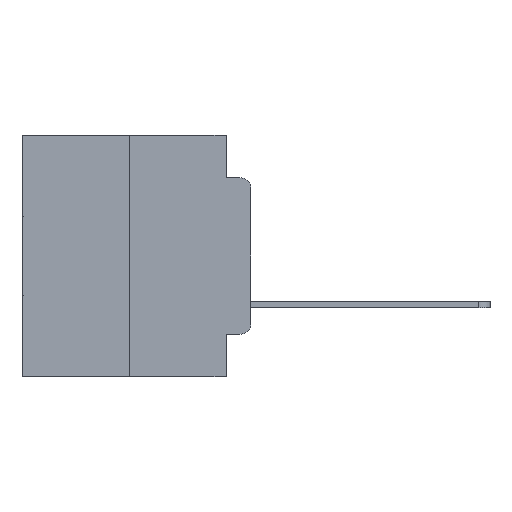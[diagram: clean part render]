
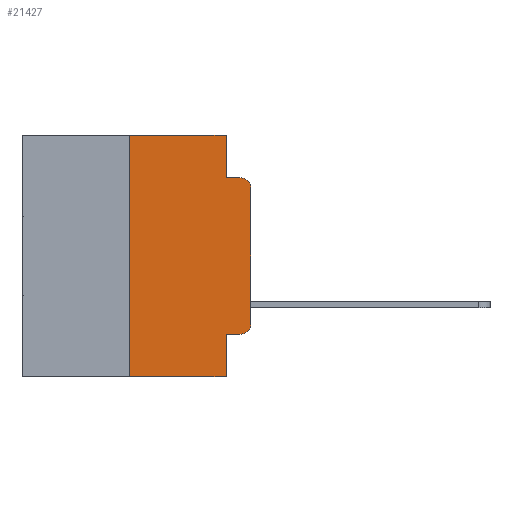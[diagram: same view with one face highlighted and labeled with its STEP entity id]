
A CAD part, left-side view. The second image highlights one B-rep face of the part: STEP entity #21427.
In plain terms, the highlighted planar face has unit normal (-1, 0, 0).
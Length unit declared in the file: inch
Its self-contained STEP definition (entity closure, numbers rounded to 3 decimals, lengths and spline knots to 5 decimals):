
#932 = VECTOR ( 'NONE', #29331, 39.37008 ) ;
#1073 = CARTESIAN_POINT ( 'NONE',  ( 0., 0.051, 0. ) ) ;
#1082 = CIRCLE ( 'NONE', #29631, 0.02 ) ;
#1406 = CARTESIAN_POINT ( 'NONE',  ( 0., 0.051, -0.4115 ) ) ;
#1834 = CARTESIAN_POINT ( 'NONE',  ( 0., 0.473, 0. ) ) ;
#1932 = VERTEX_POINT ( 'NONE', #2541 ) ;
#2098 = EDGE_CURVE ( 'NONE', #23154, #21538, #10765, .T. ) ;
#2444 = ORIENTED_EDGE ( 'NONE', *, *, #23284, .F. ) ;
#2541 = CARTESIAN_POINT ( 'NONE',  ( 0., 0.02, -0.4115 ) ) ;
#3920 = EDGE_CURVE ( 'NONE', #15514, #21538, #1082, .T. ) ;
#3952 = CARTESIAN_POINT ( 'NONE',  ( 0., 0.051, 0. ) ) ;
#4175 = DIRECTION ( 'NONE',  ( 0., 0., -1. ) ) ;
#4284 = ORIENTED_EDGE ( 'NONE', *, *, #19115, .T. ) ;
#4385 = CARTESIAN_POINT ( 'NONE',  ( 0., 0., -0.1085 ) ) ;
#5041 = LINE ( 'NONE', #1073, #9694 ) ;
#5092 = CARTESIAN_POINT ( 'NONE',  ( 0., 0.25, -0.5 ) ) ;
#5167 = EDGE_CURVE ( 'NONE', #24526, #7780, #13164, .T. ) ;
#5231 = LINE ( 'NONE', #7430, #16676 ) ;
#5801 = VECTOR ( 'NONE', #24814, 39.37008 ) ;
#5997 = EDGE_CURVE ( 'NONE', #14562, #14727, #14901, .T. ) ;
#6457 = AXIS2_PLACEMENT_3D ( 'NONE', #1834, #17892, #4175 ) ;
#6482 = EDGE_CURVE ( 'NONE', #7780, #13479, #5231, .T. ) ;
#6820 = CARTESIAN_POINT ( 'NONE',  ( 0., 0., -0.3915 ) ) ;
#6887 = DIRECTION ( 'NONE',  ( -1., 0., 0. ) ) ;
#7288 = DIRECTION ( 'NONE',  ( 0., 0., 1. ) ) ;
#7430 = CARTESIAN_POINT ( 'NONE',  ( 0., 0.473, 0. ) ) ;
#7780 = VERTEX_POINT ( 'NONE', #11738 ) ;
#7802 = ORIENTED_EDGE ( 'NONE', *, *, #6482, .F. ) ;
#8740 = CARTESIAN_POINT ( 'NONE',  ( 0., 0.473, -0.5 ) ) ;
#9685 = EDGE_CURVE ( 'NONE', #24526, #14727, #23420, .T. ) ;
#9694 = VECTOR ( 'NONE', #21288, 39.37008 ) ;
#10371 = CARTESIAN_POINT ( 'NONE',  ( 0., 0.051, -0.0885 ) ) ;
#10657 = LINE ( 'NONE', #21004, #13135 ) ;
#10765 = LINE ( 'NONE', #10371, #12912 ) ;
#11738 = CARTESIAN_POINT ( 'NONE',  ( 0., 0.25, 0. ) ) ;
#11756 = CARTESIAN_POINT ( 'NONE',  ( 0., 0.051, -0.0885 ) ) ;
#12136 = ORIENTED_EDGE ( 'NONE', *, *, #25440, .T. ) ;
#12436 = DIRECTION ( 'NONE',  ( 0., 0., -1. ) ) ;
#12912 = VECTOR ( 'NONE', #17546, 39.37008 ) ;
#13135 = VECTOR ( 'NONE', #7288, 39.37008 ) ;
#13164 = LINE ( 'NONE', #29224, #932 ) ;
#13479 = VERTEX_POINT ( 'NONE', #3952 ) ;
#13699 = CARTESIAN_POINT ( 'NONE',  ( 0., 0.02, -0.1085 ) ) ;
#13722 = ORIENTED_EDGE ( 'NONE', *, *, #28634, .T. ) ;
#13860 = DIRECTION ( 'NONE',  ( 0., 0., -1. ) ) ;
#14562 = VERTEX_POINT ( 'NONE', #21377 ) ;
#14567 = VECTOR ( 'NONE', #12436, 39.37008 ) ;
#14727 = VERTEX_POINT ( 'NONE', #27064 ) ;
#14901 = LINE ( 'NONE', #24194, #14567 ) ;
#15514 = VERTEX_POINT ( 'NONE', #4385 ) ;
#15583 = PLANE ( 'NONE',  #6457 ) ;
#16021 = DIRECTION ( 'NONE',  ( 0., 0., -1. ) ) ;
#16183 = FACE_OUTER_BOUND ( 'NONE', #27299, .T. ) ;
#16277 = CIRCLE ( 'NONE', #17492, 0.02 ) ;
#16676 = VECTOR ( 'NONE', #25785, 39.37008 ) ;
#17492 = AXIS2_PLACEMENT_3D ( 'NONE', #22825, #6887, #13860 ) ;
#17546 = DIRECTION ( 'NONE',  ( 0., -1., 0. ) ) ;
#17892 = DIRECTION ( 'NONE',  ( 1., 0., 0. ) ) ;
#19115 = EDGE_CURVE ( 'NONE', #20649, #15514, #10657, .T. ) ;
#19207 = LINE ( 'NONE', #1406, #19574 ) ;
#19574 = VECTOR ( 'NONE', #26526, 39.37008 ) ;
#20536 = ORIENTED_EDGE ( 'NONE', *, *, #9685, .T. ) ;
#20649 = VERTEX_POINT ( 'NONE', #6820 ) ;
#21004 = CARTESIAN_POINT ( 'NONE',  ( 0., 0., 0. ) ) ;
#21288 = DIRECTION ( 'NONE',  ( 0., 0., -1. ) ) ;
#21377 = CARTESIAN_POINT ( 'NONE',  ( 0., 0.051, -0.4115 ) ) ;
#21427 = ADVANCED_FACE ( 'NONE', ( #16183 ), #15583, .F. ) ;
#21538 = VERTEX_POINT ( 'NONE', #27658 ) ;
#22825 = CARTESIAN_POINT ( 'NONE',  ( 0., 0.02, -0.3915 ) ) ;
#23154 = VERTEX_POINT ( 'NONE', #11756 ) ;
#23284 = EDGE_CURVE ( 'NONE', #13479, #23154, #5041, .T. ) ;
#23420 = LINE ( 'NONE', #8740, #5801 ) ;
#23499 = ORIENTED_EDGE ( 'NONE', *, *, #2098, .F. ) ;
#24194 = CARTESIAN_POINT ( 'NONE',  ( 0., 0.051, 0. ) ) ;
#24526 = VERTEX_POINT ( 'NONE', #5092 ) ;
#24814 = DIRECTION ( 'NONE',  ( 0., -1., 0. ) ) ;
#24903 = ORIENTED_EDGE ( 'NONE', *, *, #5997, .F. ) ;
#25440 = EDGE_CURVE ( 'NONE', #14562, #1932, #19207, .T. ) ;
#25785 = DIRECTION ( 'NONE',  ( 0., -1., 0. ) ) ;
#26526 = DIRECTION ( 'NONE',  ( 0., -1., 0. ) ) ;
#26833 = ORIENTED_EDGE ( 'NONE', *, *, #3920, .T. ) ;
#27013 = ORIENTED_EDGE ( 'NONE', *, *, #5167, .F. ) ;
#27064 = CARTESIAN_POINT ( 'NONE',  ( 0., 0.051, -0.5 ) ) ;
#27299 = EDGE_LOOP ( 'NONE', ( #4284, #26833, #23499, #2444, #7802, #27013, #20536, #24903, #12136, #13722 ) ) ;
#27658 = CARTESIAN_POINT ( 'NONE',  ( 0., 0.02, -0.0885 ) ) ;
#28634 = EDGE_CURVE ( 'NONE', #1932, #20649, #16277, .T. ) ;
#29224 = CARTESIAN_POINT ( 'NONE',  ( 0., 0.25, 0. ) ) ;
#29331 = DIRECTION ( 'NONE',  ( 0., 0., 1. ) ) ;
#29631 = AXIS2_PLACEMENT_3D ( 'NONE', #13699, #29789, #16021 ) ;
#29789 = DIRECTION ( 'NONE',  ( -1., 0., 0. ) ) ;
